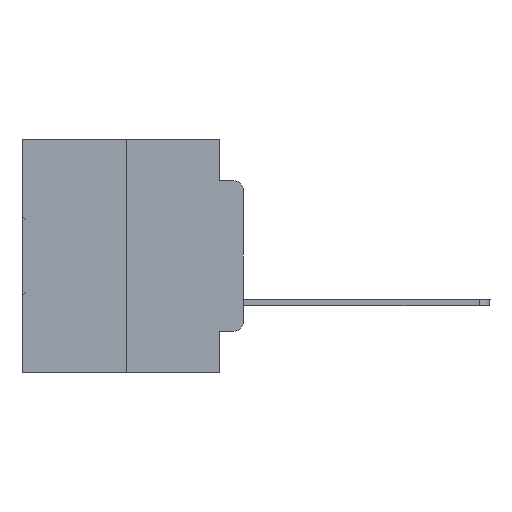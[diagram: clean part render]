
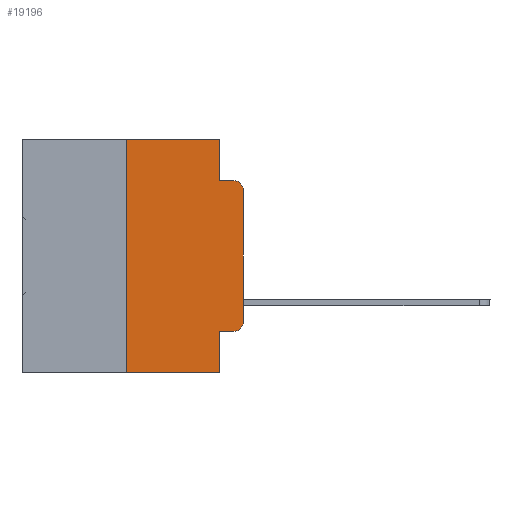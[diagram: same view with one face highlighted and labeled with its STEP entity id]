
A CAD part, left-side view. The second image highlights one B-rep face of the part: STEP entity #19196.
In plain terms, the highlighted planar face has unit normal (-1, 0, 0).
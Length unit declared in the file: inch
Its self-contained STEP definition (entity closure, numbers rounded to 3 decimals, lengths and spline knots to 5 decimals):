
#954 = CARTESIAN_POINT ( 'NONE',  ( 0., 0.051, -0.5 ) ) ;
#1124 = CARTESIAN_POINT ( 'NONE',  ( 0., 0.051, -0.4115 ) ) ;
#1713 = EDGE_CURVE ( 'NONE', #26433, #10973, #32026, .T. ) ;
#1982 = VECTOR ( 'NONE', #27296, 39.37008 ) ;
#2338 = ORIENTED_EDGE ( 'NONE', *, *, #14991, .T. ) ;
#3406 = LINE ( 'NONE', #1124, #18210 ) ;
#3587 = EDGE_CURVE ( 'NONE', #30146, #7379, #32676, .T. ) ;
#4432 = LINE ( 'NONE', #12449, #17889 ) ;
#4548 = EDGE_CURVE ( 'NONE', #13706, #19588, #4432, .T. ) ;
#4987 = ORIENTED_EDGE ( 'NONE', *, *, #20232, .T. ) ;
#5039 = DIRECTION ( 'NONE',  ( 0., -1., 0. ) ) ;
#5169 = AXIS2_PLACEMENT_3D ( 'NONE', #31755, #21277, #23902 ) ;
#5406 = CARTESIAN_POINT ( 'NONE',  ( 0., 0., -0.1085 ) ) ;
#6012 = DIRECTION ( 'NONE',  ( 0., 0., -1. ) ) ;
#7156 = CARTESIAN_POINT ( 'NONE',  ( 0., 0.051, -0.0885 ) ) ;
#7379 = VERTEX_POINT ( 'NONE', #15965 ) ;
#7781 = VECTOR ( 'NONE', #18181, 39.37008 ) ;
#8589 = ORIENTED_EDGE ( 'NONE', *, *, #3587, .F. ) ;
#9409 = VECTOR ( 'NONE', #20464, 39.37008 ) ;
#9804 = LINE ( 'NONE', #26023, #9409 ) ;
#10620 = ORIENTED_EDGE ( 'NONE', *, *, #26214, .F. ) ;
#10631 = PLANE ( 'NONE',  #5169 ) ;
#10717 = VERTEX_POINT ( 'NONE', #28172 ) ;
#10973 = VERTEX_POINT ( 'NONE', #30591 ) ;
#11962 = CARTESIAN_POINT ( 'NONE',  ( 0., 0.051, 0. ) ) ;
#12062 = CARTESIAN_POINT ( 'NONE',  ( 0., 0.02, -0.1085 ) ) ;
#12436 = CARTESIAN_POINT ( 'NONE',  ( 0., 0.25, -0.5 ) ) ;
#12449 = CARTESIAN_POINT ( 'NONE',  ( 0., 0.051, 0. ) ) ;
#12604 = VERTEX_POINT ( 'NONE', #7156 ) ;
#13287 = CARTESIAN_POINT ( 'NONE',  ( 0., 0.02, -0.4115 ) ) ;
#13572 = VECTOR ( 'NONE', #15891, 39.37008 ) ;
#13706 = VERTEX_POINT ( 'NONE', #22074 ) ;
#14549 = LINE ( 'NONE', #25176, #1982 ) ;
#14686 = DIRECTION ( 'NONE',  ( 0., 0., 1. ) ) ;
#14991 = EDGE_CURVE ( 'NONE', #13706, #26433, #3406, .T. ) ;
#15730 = AXIS2_PLACEMENT_3D ( 'NONE', #12062, #22878, #17308 ) ;
#15891 = DIRECTION ( 'NONE',  ( 0., 0., -1. ) ) ;
#15911 = ORIENTED_EDGE ( 'NONE', *, *, #4548, .F. ) ;
#15965 = CARTESIAN_POINT ( 'NONE',  ( 0., 0.25, 0. ) ) ;
#17181 = DIRECTION ( 'NONE',  ( -1., 0., 0. ) ) ;
#17308 = DIRECTION ( 'NONE',  ( 0., 0., -1. ) ) ;
#17889 = VECTOR ( 'NONE', #31138, 39.37008 ) ;
#17931 = ORIENTED_EDGE ( 'NONE', *, *, #31862, .F. ) ;
#18181 = DIRECTION ( 'NONE',  ( 0., 0., 1. ) ) ;
#18210 = VECTOR ( 'NONE', #33236, 39.37008 ) ;
#18346 = VECTOR ( 'NONE', #5039, 39.37008 ) ;
#18484 = FACE_OUTER_BOUND ( 'NONE', #19735, .T. ) ;
#18830 = CARTESIAN_POINT ( 'NONE',  ( 0., 0.051, -0.0885 ) ) ;
#19196 = ADVANCED_FACE ( 'NONE', ( #18484 ), #10631, .F. ) ;
#19343 = ORIENTED_EDGE ( 'NONE', *, *, #34021, .T. ) ;
#19562 = ORIENTED_EDGE ( 'NONE', *, *, #26752, .F. ) ;
#19588 = VERTEX_POINT ( 'NONE', #954 ) ;
#19735 = EDGE_LOOP ( 'NONE', ( #33856, #4987, #19562, #17931, #10620, #8589, #19343, #15911, #2338, #22907 ) ) ;
#20232 = EDGE_CURVE ( 'NONE', #20414, #10717, #33002, .T. ) ;
#20414 = VERTEX_POINT ( 'NONE', #5406 ) ;
#20464 = DIRECTION ( 'NONE',  ( 0., -1., 0. ) ) ;
#21198 = CARTESIAN_POINT ( 'NONE',  ( 0., 0.02, -0.3915 ) ) ;
#21277 = DIRECTION ( 'NONE',  ( 1., 0., 0. ) ) ;
#22074 = CARTESIAN_POINT ( 'NONE',  ( 0., 0.051, -0.4115 ) ) ;
#22519 = VECTOR ( 'NONE', #14686, 39.37008 ) ;
#22878 = DIRECTION ( 'NONE',  ( -1., 0., 0. ) ) ;
#22907 = ORIENTED_EDGE ( 'NONE', *, *, #1713, .T. ) ;
#23404 = CARTESIAN_POINT ( 'NONE',  ( 0., 0., 0. ) ) ;
#23902 = DIRECTION ( 'NONE',  ( 0., 0., -1. ) ) ;
#25176 = CARTESIAN_POINT ( 'NONE',  ( 0., 0.473, -0.5 ) ) ;
#26023 = CARTESIAN_POINT ( 'NONE',  ( 0., 0.473, 0. ) ) ;
#26214 = EDGE_CURVE ( 'NONE', #7379, #28808, #9804, .T. ) ;
#26433 = VERTEX_POINT ( 'NONE', #13287 ) ;
#26752 = EDGE_CURVE ( 'NONE', #12604, #10717, #29289, .T. ) ;
#27296 = DIRECTION ( 'NONE',  ( 0., -1., 0. ) ) ;
#28172 = CARTESIAN_POINT ( 'NONE',  ( 0., 0.02, -0.0885 ) ) ;
#28808 = VERTEX_POINT ( 'NONE', #11962 ) ;
#28963 = CARTESIAN_POINT ( 'NONE',  ( 0., 0.051, 0. ) ) ;
#29066 = EDGE_CURVE ( 'NONE', #10973, #20414, #32522, .T. ) ;
#29289 = LINE ( 'NONE', #18830, #18346 ) ;
#30146 = VERTEX_POINT ( 'NONE', #12436 ) ;
#30217 = CARTESIAN_POINT ( 'NONE',  ( 0., 0.25, 0. ) ) ;
#30591 = CARTESIAN_POINT ( 'NONE',  ( 0., 0., -0.3915 ) ) ;
#31138 = DIRECTION ( 'NONE',  ( 0., 0., -1. ) ) ;
#31755 = CARTESIAN_POINT ( 'NONE',  ( 0., 0.473, 0. ) ) ;
#31862 = EDGE_CURVE ( 'NONE', #28808, #12604, #32292, .T. ) ;
#32026 = CIRCLE ( 'NONE', #33148, 0.02 ) ;
#32292 = LINE ( 'NONE', #28963, #13572 ) ;
#32522 = LINE ( 'NONE', #23404, #7781 ) ;
#32676 = LINE ( 'NONE', #30217, #22519 ) ;
#33002 = CIRCLE ( 'NONE', #15730, 0.02 ) ;
#33148 = AXIS2_PLACEMENT_3D ( 'NONE', #21198, #17181, #6012 ) ;
#33236 = DIRECTION ( 'NONE',  ( 0., -1., 0. ) ) ;
#33856 = ORIENTED_EDGE ( 'NONE', *, *, #29066, .T. ) ;
#34021 = EDGE_CURVE ( 'NONE', #30146, #19588, #14549, .T. ) ;
